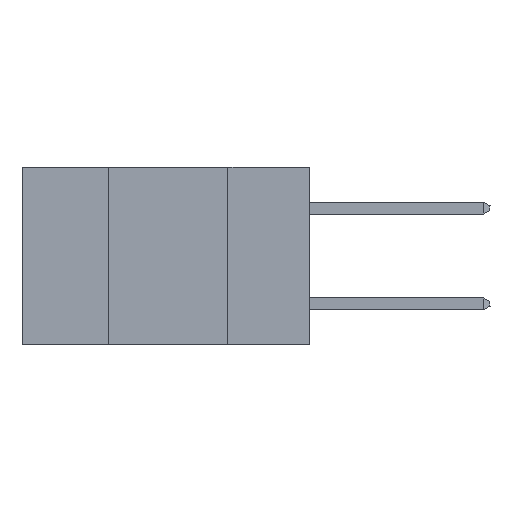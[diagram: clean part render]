
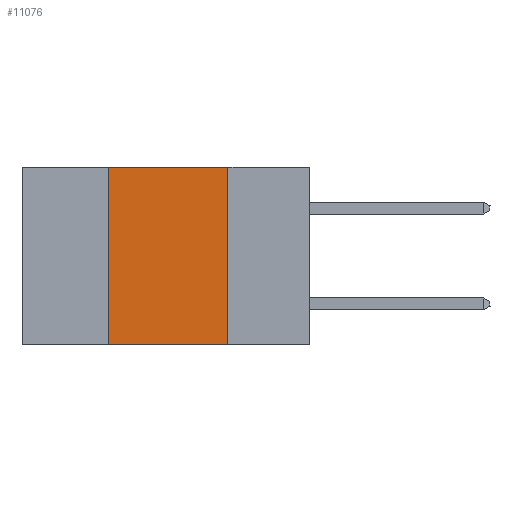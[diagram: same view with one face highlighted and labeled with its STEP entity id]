
A CAD part, left-side view. The second image highlights one B-rep face of the part: STEP entity #11076.
In plain terms, the highlighted planar face has unit normal (-1, 0, 0).
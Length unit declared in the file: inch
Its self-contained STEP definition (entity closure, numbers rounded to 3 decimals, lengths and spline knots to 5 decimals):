
#383 = CARTESIAN_POINT ( 'NONE',  ( 0., 0.17, -0.37 ) ) ;
#616 = VERTEX_POINT ( 'NONE', #20459 ) ;
#627 = DIRECTION ( 'NONE',  ( 1., 0., 0. ) ) ;
#1614 = CARTESIAN_POINT ( 'NONE',  ( 0., 0.42, 0. ) ) ;
#1699 = DIRECTION ( 'NONE',  ( 0., -1., 0. ) ) ;
#1753 = DIRECTION ( 'NONE',  ( 0., 0., 1. ) ) ;
#1948 = VECTOR ( 'NONE', #1753, 39.37008 ) ;
#2711 = EDGE_CURVE ( 'NONE', #16196, #13282, #6231, .T. ) ;
#2847 = CARTESIAN_POINT ( 'NONE',  ( 0., 0.6, 0. ) ) ;
#2981 = VERTEX_POINT ( 'NONE', #383 ) ;
#3548 = ORIENTED_EDGE ( 'NONE', *, *, #18184, .F. ) ;
#3889 = VECTOR ( 'NONE', #18957, 39.37008 ) ;
#4860 = EDGE_CURVE ( 'NONE', #616, #2981, #16120, .T. ) ;
#5858 = CARTESIAN_POINT ( 'NONE',  ( 0., 0.42, -0.37 ) ) ;
#6231 = LINE ( 'NONE', #1614, #1948 ) ;
#7923 = CARTESIAN_POINT ( 'NONE',  ( 0., 0.17, 0. ) ) ;
#8148 = EDGE_CURVE ( 'NONE', #16196, #2981, #20090, .T. ) ;
#8736 = PLANE ( 'NONE',  #17305 ) ;
#8844 = EDGE_LOOP ( 'NONE', ( #10407, #3548, #14331, #17136 ) ) ;
#9361 = DIRECTION ( 'NONE',  ( 0., -1., 0. ) ) ;
#9784 = CARTESIAN_POINT ( 'NONE',  ( 0., 0.6, -0.37 ) ) ;
#10407 = ORIENTED_EDGE ( 'NONE', *, *, #4860, .F. ) ;
#11076 = ADVANCED_FACE ( 'NONE', ( #20005 ), #8736, .F. ) ;
#11773 = VECTOR ( 'NONE', #1699, 39.37008 ) ;
#11948 = DIRECTION ( 'NONE',  ( 0., 0., -1. ) ) ;
#13282 = VERTEX_POINT ( 'NONE', #13691 ) ;
#13691 = CARTESIAN_POINT ( 'NONE',  ( 0., 0.42, 0. ) ) ;
#14331 = ORIENTED_EDGE ( 'NONE', *, *, #2711, .F. ) ;
#16120 = LINE ( 'NONE', #7923, #3889 ) ;
#16196 = VERTEX_POINT ( 'NONE', #5858 ) ;
#17136 = ORIENTED_EDGE ( 'NONE', *, *, #8148, .T. ) ;
#17205 = LINE ( 'NONE', #2847, #18178 ) ;
#17305 = AXIS2_PLACEMENT_3D ( 'NONE', #19748, #627, #11948 ) ;
#18178 = VECTOR ( 'NONE', #9361, 39.37008 ) ;
#18184 = EDGE_CURVE ( 'NONE', #13282, #616, #17205, .T. ) ;
#18957 = DIRECTION ( 'NONE',  ( 0., 0., -1. ) ) ;
#19748 = CARTESIAN_POINT ( 'NONE',  ( 0., 0.6, 0. ) ) ;
#20005 = FACE_OUTER_BOUND ( 'NONE', #8844, .T. ) ;
#20090 = LINE ( 'NONE', #9784, #11773 ) ;
#20459 = CARTESIAN_POINT ( 'NONE',  ( 0., 0.17, 0. ) ) ;
